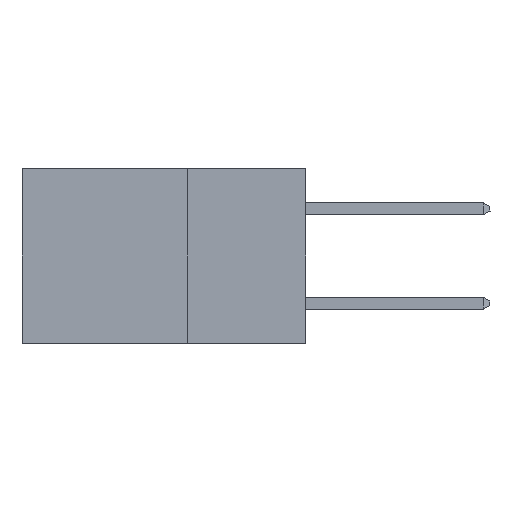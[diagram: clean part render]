
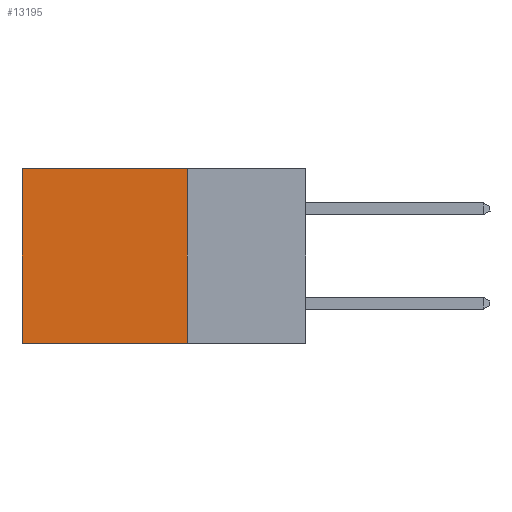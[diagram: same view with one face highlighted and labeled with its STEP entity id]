
A CAD part, left-side view. The second image highlights one B-rep face of the part: STEP entity #13195.
In plain terms, the highlighted planar face has unit normal (-1, 0, 0).
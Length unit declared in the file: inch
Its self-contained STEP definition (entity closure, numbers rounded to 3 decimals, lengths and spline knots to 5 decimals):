
#362 = EDGE_CURVE ( 'NONE', #9181, #2285, #907, .T. ) ;
#874 = EDGE_LOOP ( 'NONE', ( #2587, #12124, #12782, #8711 ) ) ;
#907 = LINE ( 'NONE', #9539, #13024 ) ;
#2285 = VERTEX_POINT ( 'NONE', #14996 ) ;
#2501 = CARTESIAN_POINT ( 'NONE',  ( 0.298, 0.25, 0. ) ) ;
#2587 = ORIENTED_EDGE ( 'NONE', *, *, #362, .T. ) ;
#3280 = CARTESIAN_POINT ( 'NONE',  ( 0.298, 0.25, 0. ) ) ;
#3718 = DIRECTION ( 'NONE',  ( 1., 0., 0. ) ) ;
#4198 = EDGE_CURVE ( 'NONE', #6915, #7017, #9383, .T. ) ;
#4205 = VECTOR ( 'NONE', #4261, 39.37008 ) ;
#4261 = DIRECTION ( 'NONE',  ( 0., 1., 0. ) ) ;
#6194 = VECTOR ( 'NONE', #13394, 39.37008 ) ;
#6211 = CARTESIAN_POINT ( 'NONE',  ( 0.298, 0.6, 0. ) ) ;
#6468 = EDGE_CURVE ( 'NONE', #6915, #9181, #7807, .T. ) ;
#6915 = VERTEX_POINT ( 'NONE', #2501 ) ;
#7017 = VERTEX_POINT ( 'NONE', #14686 ) ;
#7807 = LINE ( 'NONE', #14100, #4205 ) ;
#7954 = FACE_OUTER_BOUND ( 'NONE', #874, .T. ) ;
#8260 = VECTOR ( 'NONE', #15450, 39.37008 ) ;
#8711 = ORIENTED_EDGE ( 'NONE', *, *, #6468, .T. ) ;
#9012 = LINE ( 'NONE', #12260, #6194 ) ;
#9166 = EDGE_CURVE ( 'NONE', #7017, #2285, #9012, .T. ) ;
#9181 = VERTEX_POINT ( 'NONE', #6211 ) ;
#9383 = LINE ( 'NONE', #3280, #8260 ) ;
#9539 = CARTESIAN_POINT ( 'NONE',  ( 0.298, 0.6, 0. ) ) ;
#9582 = AXIS2_PLACEMENT_3D ( 'NONE', #13302, #3718, #10918 ) ;
#10918 = DIRECTION ( 'NONE',  ( 0., 0., -1. ) ) ;
#11861 = DIRECTION ( 'NONE',  ( 0., 0., -1. ) ) ;
#12124 = ORIENTED_EDGE ( 'NONE', *, *, #9166, .F. ) ;
#12260 = CARTESIAN_POINT ( 'NONE',  ( 0.298, 0.25, -0.37 ) ) ;
#12782 = ORIENTED_EDGE ( 'NONE', *, *, #4198, .F. ) ;
#13024 = VECTOR ( 'NONE', #11861, 39.37008 ) ;
#13195 = ADVANCED_FACE ( 'NONE', ( #7954 ), #15680, .F. ) ;
#13302 = CARTESIAN_POINT ( 'NONE',  ( 0.298, 0.25, 0. ) ) ;
#13394 = DIRECTION ( 'NONE',  ( 0., 1., 0. ) ) ;
#14100 = CARTESIAN_POINT ( 'NONE',  ( 0.298, 0.25, 0. ) ) ;
#14686 = CARTESIAN_POINT ( 'NONE',  ( 0.298, 0.25, -0.37 ) ) ;
#14996 = CARTESIAN_POINT ( 'NONE',  ( 0.298, 0.6, -0.37 ) ) ;
#15450 = DIRECTION ( 'NONE',  ( 0., 0., -1. ) ) ;
#15680 = PLANE ( 'NONE',  #9582 ) ;
